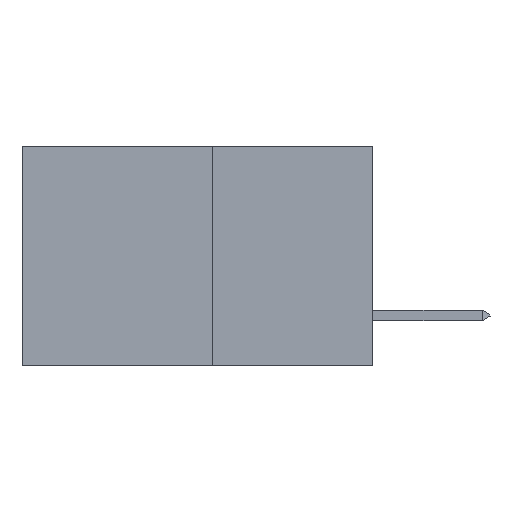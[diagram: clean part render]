
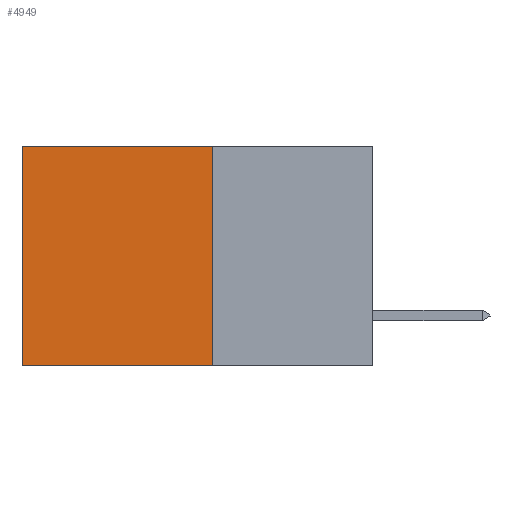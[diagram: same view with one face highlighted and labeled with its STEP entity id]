
A CAD part, left-side view. The second image highlights one B-rep face of the part: STEP entity #4949.
In plain terms, the highlighted planar face has unit normal (-1, 0, 0).
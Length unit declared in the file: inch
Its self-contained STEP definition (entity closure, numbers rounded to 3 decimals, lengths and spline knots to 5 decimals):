
#751 = AXIS2_PLACEMENT_3D ( 'NONE', #7006, #6928, #6909 ) ;
#2174 = CARTESIAN_POINT ( 'NONE',  ( 0.277, 0.27, 0. ) ) ;
#2621 = VECTOR ( 'NONE', #9107, 39.37008 ) ;
#2751 = CARTESIAN_POINT ( 'NONE',  ( 0.277, 0.59, -0.37 ) ) ;
#2762 = VERTEX_POINT ( 'NONE', #12568 ) ;
#3602 = EDGE_CURVE ( 'NONE', #12013, #2762, #10215, .T. ) ;
#3762 = CARTESIAN_POINT ( 'NONE',  ( 0.277, 0.27, 0. ) ) ;
#4910 = CARTESIAN_POINT ( 'NONE',  ( 0.277, 0.59, 0. ) ) ;
#4913 = ORIENTED_EDGE ( 'NONE', *, *, #7526, .T. ) ;
#4914 = DIRECTION ( 'NONE',  ( 0., 0., -1. ) ) ;
#4949 = ADVANCED_FACE ( 'NONE', ( #14884 ), #6943, .F. ) ;
#5073 = CARTESIAN_POINT ( 'NONE',  ( 0.277, 0.27, -0.37 ) ) ;
#5255 = VERTEX_POINT ( 'NONE', #4910 ) ;
#5271 = ORIENTED_EDGE ( 'NONE', *, *, #13477, .F. ) ;
#6363 = ORIENTED_EDGE ( 'NONE', *, *, #3602, .F. ) ;
#6909 = DIRECTION ( 'NONE',  ( 0., 0., -1. ) ) ;
#6928 = DIRECTION ( 'NONE',  ( 1., 0., 0. ) ) ;
#6943 = PLANE ( 'NONE',  #751 ) ;
#7005 = VECTOR ( 'NONE', #4914, 39.37008 ) ;
#7006 = CARTESIAN_POINT ( 'NONE',  ( 0.277, 0.27, -0.37 ) ) ;
#7526 = EDGE_CURVE ( 'NONE', #5255, #12370, #11020, .T. ) ;
#7666 = VECTOR ( 'NONE', #10581, 39.37008 ) ;
#7826 = VECTOR ( 'NONE', #8424, 39.37008 ) ;
#8424 = DIRECTION ( 'NONE',  ( 0., 0., -1. ) ) ;
#8724 = CARTESIAN_POINT ( 'NONE',  ( 0.277, 0.59, -0.37 ) ) ;
#9107 = DIRECTION ( 'NONE',  ( 0., 1., 0. ) ) ;
#9393 = CARTESIAN_POINT ( 'NONE',  ( 0.277, 0.27, -0.37 ) ) ;
#10215 = LINE ( 'NONE', #5073, #7005 ) ;
#10581 = DIRECTION ( 'NONE',  ( 0., 1., 0. ) ) ;
#11020 = LINE ( 'NONE', #8724, #7826 ) ;
#11616 = LINE ( 'NONE', #2174, #2621 ) ;
#11872 = EDGE_LOOP ( 'NONE', ( #4913, #5271, #6363, #12709 ) ) ;
#12013 = VERTEX_POINT ( 'NONE', #3762 ) ;
#12370 = VERTEX_POINT ( 'NONE', #2751 ) ;
#12568 = CARTESIAN_POINT ( 'NONE',  ( 0.277, 0.27, -0.37 ) ) ;
#12709 = ORIENTED_EDGE ( 'NONE', *, *, #14026, .T. ) ;
#13477 = EDGE_CURVE ( 'NONE', #2762, #12370, #14286, .T. ) ;
#14026 = EDGE_CURVE ( 'NONE', #12013, #5255, #11616, .T. ) ;
#14286 = LINE ( 'NONE', #9393, #7666 ) ;
#14884 = FACE_OUTER_BOUND ( 'NONE', #11872, .T. ) ;
